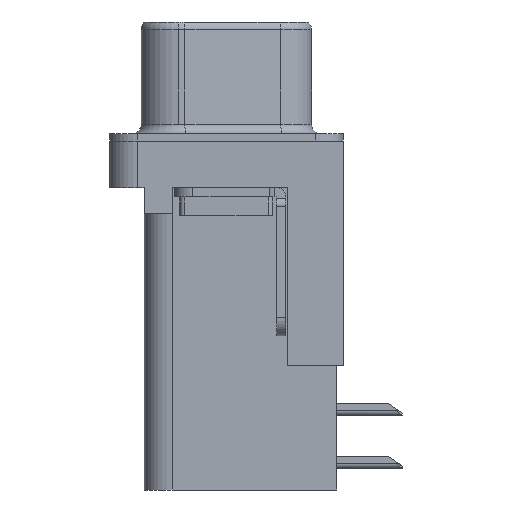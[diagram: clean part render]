
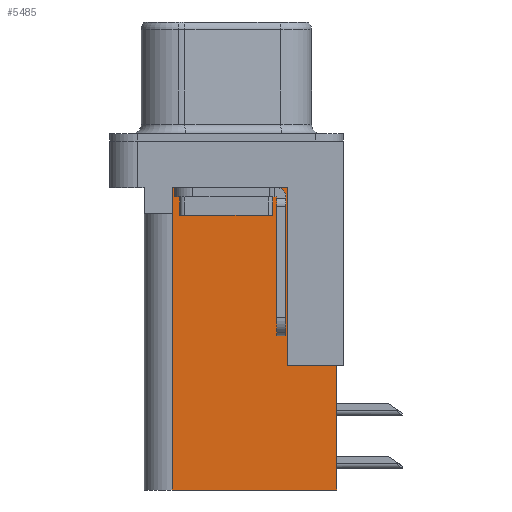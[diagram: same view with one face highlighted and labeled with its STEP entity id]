
A CAD part, left-side view. The second image highlights one B-rep face of the part: STEP entity #5485.
In plain terms, the highlighted planar face has unit normal (-1, 0, 0).
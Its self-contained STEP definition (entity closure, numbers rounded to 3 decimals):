
#24 = CARTESIAN_POINT ( 'NONE',  ( 3.79, -3.295, -12.05 ) ) ;
#181 = CARTESIAN_POINT ( 'NONE',  ( 3.79, 2.925, -18.76 ) ) ;
#216 = EDGE_CURVE ( 'NONE', #7131, #569, #7073, .T. ) ;
#237 = EDGE_CURVE ( 'NONE', #2925, #7131, #7020, .T. ) ;
#520 = CARTESIAN_POINT ( 'NONE',  ( 3.79, 2.925, -3.9 ) ) ;
#569 = VERTEX_POINT ( 'NONE', #520 ) ;
#892 = CARTESIAN_POINT ( 'NONE',  ( 3.79, -3.295, -2.5 ) ) ;
#1179 = LINE ( 'NONE', #6471, #6273 ) ;
#1343 = VECTOR ( 'NONE', #7675, 1000. ) ;
#1862 = VECTOR ( 'NONE', #2514, 1000. ) ;
#1899 = ORIENTED_EDGE ( 'NONE', *, *, #5495, .F. ) ;
#2227 = CARTESIAN_POINT ( 'NONE',  ( 3.79, 2.895, -3.9 ) ) ;
#2506 = DIRECTION ( 'NONE',  ( 0., 1., 0. ) ) ;
#2514 = DIRECTION ( 'NONE',  ( 0., 0., 1. ) ) ;
#2582 = VERTEX_POINT ( 'NONE', #11854 ) ;
#2838 = DIRECTION ( 'NONE',  ( 0., 0., 1. ) ) ;
#2925 = VERTEX_POINT ( 'NONE', #11031 ) ;
#2937 = CARTESIAN_POINT ( 'NONE',  ( 3.79, -3.295, -18.76 ) ) ;
#3359 = EDGE_CURVE ( 'NONE', #11468, #2925, #5671, .T. ) ;
#4113 = LINE ( 'NONE', #2937, #6776 ) ;
#5025 = EDGE_CURVE ( 'NONE', #2582, #7856, #1179, .T. ) ;
#5120 = EDGE_CURVE ( 'NONE', #7856, #10382, #7414, .T. ) ;
#5146 = EDGE_CURVE ( 'NONE', #5448, #11468, #4113, .T. ) ;
#5233 = EDGE_CURVE ( 'NONE', #2582, #5448, #8211, .T. ) ;
#5448 = VERTEX_POINT ( 'NONE', #24 ) ;
#5479 = CARTESIAN_POINT ( 'NONE',  ( 3.79, 2.925, -18.76 ) ) ;
#5485 = ADVANCED_FACE ( 'NONE', ( #13368 ), #10181, .F. ) ;
#5495 = EDGE_CURVE ( 'NONE', #10382, #569, #11295, .T. ) ;
#5646 = DIRECTION ( 'NONE',  ( 0., 0., -1. ) ) ;
#5671 = LINE ( 'NONE', #6895, #10896 ) ;
#5766 = CARTESIAN_POINT ( 'NONE',  ( 3.79, 0., -3.9 ) ) ;
#5998 = CARTESIAN_POINT ( 'NONE',  ( 3.79, -3.295, -18.76 ) ) ;
#6044 = DIRECTION ( 'NONE',  ( 1., 0., 0. ) ) ;
#6072 = DIRECTION ( 'NONE',  ( 0., 1., 0. ) ) ;
#6273 = VECTOR ( 'NONE', #5646, 1000. ) ;
#6471 = CARTESIAN_POINT ( 'NONE',  ( 3.79, -5.925, -2. ) ) ;
#6556 = ORIENTED_EDGE ( 'NONE', *, *, #5146, .T. ) ;
#6776 = VECTOR ( 'NONE', #2838, 1000. ) ;
#6895 = CARTESIAN_POINT ( 'NONE',  ( 3.79, -3.295, -2.5 ) ) ;
#6999 = VECTOR ( 'NONE', #7710, 1000. ) ;
#7020 = LINE ( 'NONE', #7295, #6999 ) ;
#7063 = VECTOR ( 'NONE', #6072, 1000. ) ;
#7073 = LINE ( 'NONE', #5766, #7063 ) ;
#7131 = VERTEX_POINT ( 'NONE', #2227 ) ;
#7295 = CARTESIAN_POINT ( 'NONE',  ( 3.79, 2.895, -3.9 ) ) ;
#7414 = LINE ( 'NONE', #8260, #1343 ) ;
#7675 = DIRECTION ( 'NONE',  ( 0., 1., 0. ) ) ;
#7710 = DIRECTION ( 'NONE',  ( 0., 0., -1. ) ) ;
#7856 = VERTEX_POINT ( 'NONE', #10386 ) ;
#7875 = EDGE_LOOP ( 'NONE', ( #12962, #12642, #9862, #1899, #12820, #13168, #9672, #6556 ) ) ;
#8211 = LINE ( 'NONE', #12800, #13380 ) ;
#8260 = CARTESIAN_POINT ( 'NONE',  ( 3.79, -3.295, -18.76 ) ) ;
#9672 = ORIENTED_EDGE ( 'NONE', *, *, #5233, .T. ) ;
#9862 = ORIENTED_EDGE ( 'NONE', *, *, #216, .T. ) ;
#10181 = PLANE ( 'NONE',  #11447 ) ;
#10382 = VERTEX_POINT ( 'NONE', #5479 ) ;
#10386 = CARTESIAN_POINT ( 'NONE',  ( 3.79, -5.925, -18.76 ) ) ;
#10896 = VECTOR ( 'NONE', #2506, 1000. ) ;
#11031 = CARTESIAN_POINT ( 'NONE',  ( 3.79, 2.895, -2.5 ) ) ;
#11295 = LINE ( 'NONE', #181, #1862 ) ;
#11447 = AXIS2_PLACEMENT_3D ( 'NONE', #5998, #6044, #13265 ) ;
#11468 = VERTEX_POINT ( 'NONE', #892 ) ;
#11854 = CARTESIAN_POINT ( 'NONE',  ( 3.79, -5.925, -12.05 ) ) ;
#12642 = ORIENTED_EDGE ( 'NONE', *, *, #237, .T. ) ;
#12748 = DIRECTION ( 'NONE',  ( 0., 1., 0. ) ) ;
#12800 = CARTESIAN_POINT ( 'NONE',  ( 3.79, -6.295, -12.05 ) ) ;
#12820 = ORIENTED_EDGE ( 'NONE', *, *, #5120, .F. ) ;
#12962 = ORIENTED_EDGE ( 'NONE', *, *, #3359, .T. ) ;
#13168 = ORIENTED_EDGE ( 'NONE', *, *, #5025, .F. ) ;
#13265 = DIRECTION ( 'NONE',  ( 0., 1., 0. ) ) ;
#13368 = FACE_OUTER_BOUND ( 'NONE', #7875, .T. ) ;
#13380 = VECTOR ( 'NONE', #12748, 1000. ) ;
